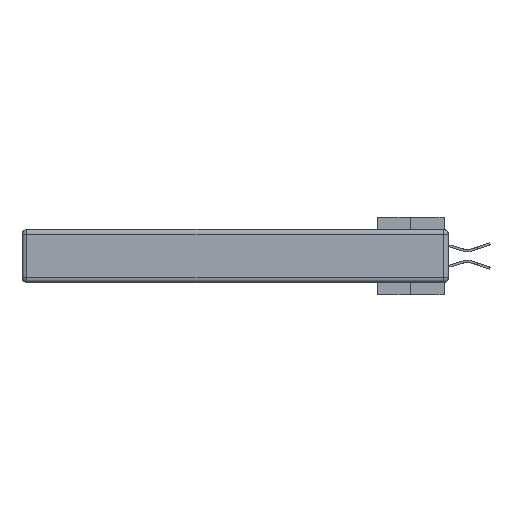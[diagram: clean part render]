
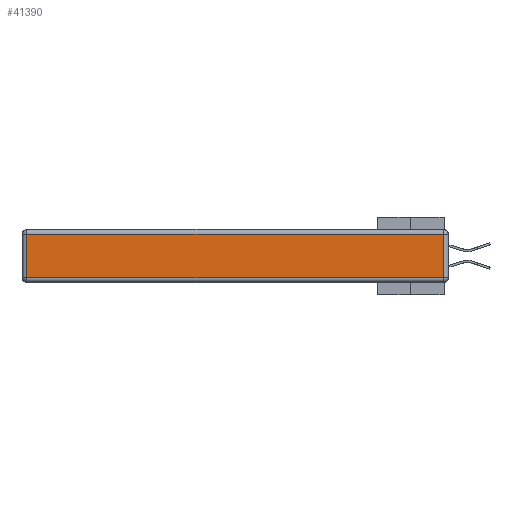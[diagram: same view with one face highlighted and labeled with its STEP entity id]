
A CAD part, left-side view. The second image highlights one B-rep face of the part: STEP entity #41390.
In plain terms, the highlighted planar face has unit normal (-1, 0, 0).
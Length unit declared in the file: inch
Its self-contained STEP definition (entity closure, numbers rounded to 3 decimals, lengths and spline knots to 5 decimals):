
#143 = CARTESIAN_POINT ( 'NONE',  ( 0., 2.72, -0.313 ) ) ;
#2110 = VERTEX_POINT ( 'NONE', #23754 ) ;
#2656 = DIRECTION ( 'NONE',  ( 0., 1., 0. ) ) ;
#4624 = PLANE ( 'NONE',  #13357 ) ;
#4973 = FACE_OUTER_BOUND ( 'NONE', #33450, .T. ) ;
#9909 = ORIENTED_EDGE ( 'NONE', *, *, #40178, .T. ) ;
#11638 = VECTOR ( 'NONE', #27278, 39.37008 ) ;
#11988 = EDGE_CURVE ( 'NONE', #40061, #2110, #38735, .T. ) ;
#13092 = VERTEX_POINT ( 'NONE', #143 ) ;
#13357 = AXIS2_PLACEMENT_3D ( 'NONE', #30636, #27385, #40742 ) ;
#13726 = LINE ( 'NONE', #37385, #21363 ) ;
#17286 = LINE ( 'NONE', #29996, #11638 ) ;
#18093 = CARTESIAN_POINT ( 'NONE',  ( 0., 0., -0.313 ) ) ;
#20810 = DIRECTION ( 'NONE',  ( 0., 0., 1. ) ) ;
#21095 = DIRECTION ( 'NONE',  ( 0., -1., 0. ) ) ;
#21325 = ORIENTED_EDGE ( 'NONE', *, *, #11988, .T. ) ;
#21363 = VECTOR ( 'NONE', #20810, 39.37008 ) ;
#22259 = CARTESIAN_POINT ( 'NONE',  ( 0., 0.03, -0.03 ) ) ;
#23589 = LINE ( 'NONE', #18093, #38352 ) ;
#23754 = CARTESIAN_POINT ( 'NONE',  ( 0., 2.72, -0.03 ) ) ;
#24199 = ORIENTED_EDGE ( 'NONE', *, *, #36612, .T. ) ;
#27278 = DIRECTION ( 'NONE',  ( 0., 0., -1. ) ) ;
#27385 = DIRECTION ( 'NONE',  ( -1., 0., 0. ) ) ;
#29996 = CARTESIAN_POINT ( 'NONE',  ( 0., 2.72, -0.343 ) ) ;
#30383 = ORIENTED_EDGE ( 'NONE', *, *, #37236, .T. ) ;
#30636 = CARTESIAN_POINT ( 'NONE',  ( 0., 0., -0.343 ) ) ;
#33450 = EDGE_LOOP ( 'NONE', ( #9909, #30383, #21325, #24199 ) ) ;
#34166 = VERTEX_POINT ( 'NONE', #37336 ) ;
#34460 = CARTESIAN_POINT ( 'NONE',  ( 0., 2.75, -0.03 ) ) ;
#36612 = EDGE_CURVE ( 'NONE', #2110, #13092, #17286, .T. ) ;
#37236 = EDGE_CURVE ( 'NONE', #34166, #40061, #13726, .T. ) ;
#37336 = CARTESIAN_POINT ( 'NONE',  ( 0., 0.03, -0.313 ) ) ;
#37385 = CARTESIAN_POINT ( 'NONE',  ( 0., 0.03, -0.343 ) ) ;
#38352 = VECTOR ( 'NONE', #21095, 39.37008 ) ;
#38735 = LINE ( 'NONE', #34460, #39261 ) ;
#39261 = VECTOR ( 'NONE', #2656, 39.37008 ) ;
#40061 = VERTEX_POINT ( 'NONE', #22259 ) ;
#40178 = EDGE_CURVE ( 'NONE', #13092, #34166, #23589, .T. ) ;
#40742 = DIRECTION ( 'NONE',  ( 0., 0., 1. ) ) ;
#41390 = ADVANCED_FACE ( 'NONE', ( #4973 ), #4624, .T. ) ;
